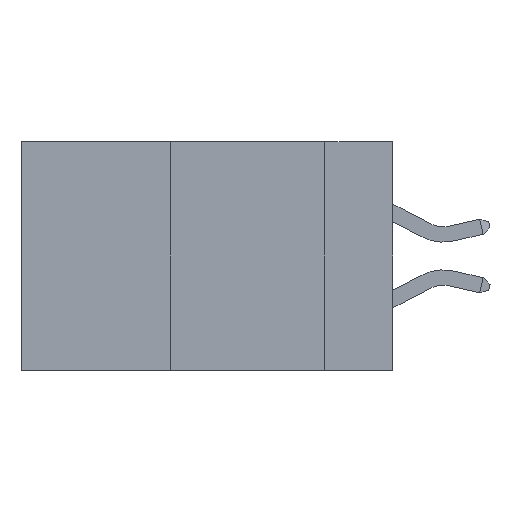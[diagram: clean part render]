
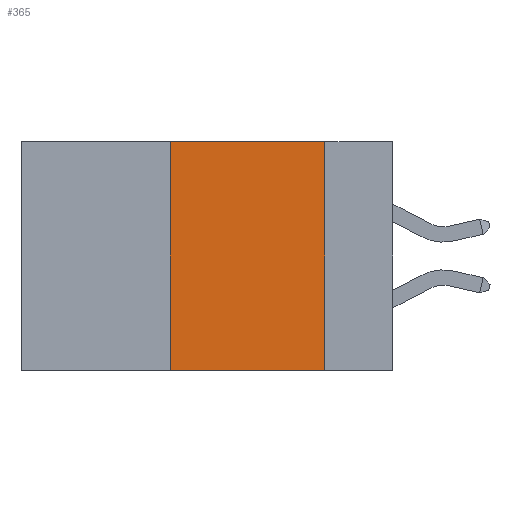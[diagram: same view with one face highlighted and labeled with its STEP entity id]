
A CAD part, left-side view. The second image highlights one B-rep face of the part: STEP entity #365.
In plain terms, the highlighted planar face has unit normal (-1, 0, 0).
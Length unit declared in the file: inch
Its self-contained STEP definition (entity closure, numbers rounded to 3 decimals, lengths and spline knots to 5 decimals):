
#186 = EDGE_CURVE ( 'NONE', #26841, #23340, #18464, .T. ) ;
#327 = CARTESIAN_POINT ( 'NONE',  ( 0., 0.36, 0. ) ) ;
#365 = ADVANCED_FACE ( 'NONE', ( #7485 ), #20952, .F. ) ;
#2173 = EDGE_CURVE ( 'NONE', #21152, #26841, #15793, .T. ) ;
#2440 = DIRECTION ( 'NONE',  ( 1., 0., 0. ) ) ;
#3551 = DIRECTION ( 'NONE',  ( 0., -1., 0. ) ) ;
#3904 = VECTOR ( 'NONE', #22726, 39.37008 ) ;
#4210 = DIRECTION ( 'NONE',  ( 0., 0., -1. ) ) ;
#5612 = EDGE_LOOP ( 'NONE', ( #11606, #13624, #17300, #16581 ) ) ;
#7485 = FACE_OUTER_BOUND ( 'NONE', #5612, .T. ) ;
#11606 = ORIENTED_EDGE ( 'NONE', *, *, #27474, .F. ) ;
#11964 = CARTESIAN_POINT ( 'NONE',  ( 0., 0.6, 0. ) ) ;
#12824 = AXIS2_PLACEMENT_3D ( 'NONE', #18807, #2440, #21543 ) ;
#13624 = ORIENTED_EDGE ( 'NONE', *, *, #186, .F. ) ;
#15274 = VECTOR ( 'NONE', #4210, 39.37008 ) ;
#15793 = LINE ( 'NONE', #327, #26648 ) ;
#16345 = VECTOR ( 'NONE', #3551, 39.37008 ) ;
#16581 = ORIENTED_EDGE ( 'NONE', *, *, #29736, .T. ) ;
#17300 = ORIENTED_EDGE ( 'NONE', *, *, #2173, .F. ) ;
#17681 = CARTESIAN_POINT ( 'NONE',  ( 0., 0.6, -0.37 ) ) ;
#18000 = CARTESIAN_POINT ( 'NONE',  ( 0., 0.36, -0.37 ) ) ;
#18350 = CARTESIAN_POINT ( 'NONE',  ( 0., 0.36, 0. ) ) ;
#18464 = LINE ( 'NONE', #11964, #3904 ) ;
#18807 = CARTESIAN_POINT ( 'NONE',  ( 0., 0.6, 0. ) ) ;
#20952 = PLANE ( 'NONE',  #12824 ) ;
#21152 = VERTEX_POINT ( 'NONE', #18000 ) ;
#21304 = CARTESIAN_POINT ( 'NONE',  ( 0., 0.11, 0. ) ) ;
#21543 = DIRECTION ( 'NONE',  ( 0., 0., -1. ) ) ;
#21700 = VERTEX_POINT ( 'NONE', #26171 ) ;
#22726 = DIRECTION ( 'NONE',  ( 0., -1., 0. ) ) ;
#23340 = VERTEX_POINT ( 'NONE', #21304 ) ;
#23967 = DIRECTION ( 'NONE',  ( 0., 0., 1. ) ) ;
#23969 = LINE ( 'NONE', #17681, #16345 ) ;
#25047 = CARTESIAN_POINT ( 'NONE',  ( 0., 0.11, 0. ) ) ;
#26171 = CARTESIAN_POINT ( 'NONE',  ( 0., 0.11, -0.37 ) ) ;
#26648 = VECTOR ( 'NONE', #23967, 39.37008 ) ;
#26841 = VERTEX_POINT ( 'NONE', #18350 ) ;
#27474 = EDGE_CURVE ( 'NONE', #23340, #21700, #28692, .T. ) ;
#28692 = LINE ( 'NONE', #25047, #15274 ) ;
#29736 = EDGE_CURVE ( 'NONE', #21152, #21700, #23969, .T. ) ;
